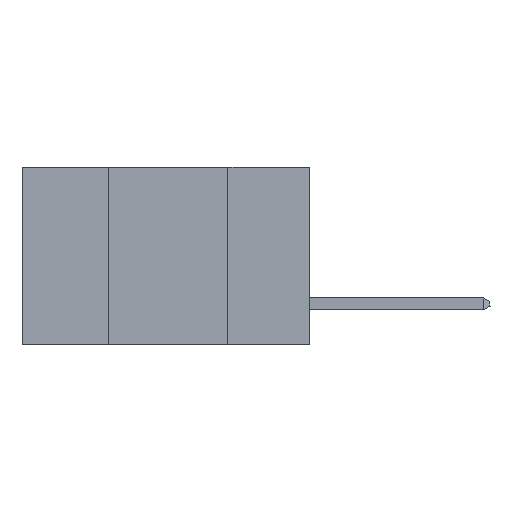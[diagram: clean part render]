
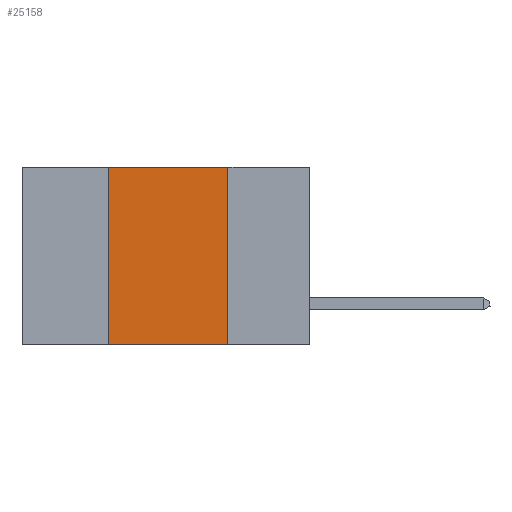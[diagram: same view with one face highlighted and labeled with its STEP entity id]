
A CAD part, left-side view. The second image highlights one B-rep face of the part: STEP entity #25158.
In plain terms, the highlighted planar face has unit normal (-1, 0, 0).
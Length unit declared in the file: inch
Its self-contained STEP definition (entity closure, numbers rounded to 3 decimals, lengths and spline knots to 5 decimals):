
#831 = DIRECTION ( 'NONE',  ( 0., 0., 1. ) ) ;
#963 = LINE ( 'NONE', #11146, #35582 ) ;
#2175 = ORIENTED_EDGE ( 'NONE', *, *, #39375, .F. ) ;
#4394 = EDGE_CURVE ( 'NONE', #23664, #35601, #20117, .T. ) ;
#5021 = ORIENTED_EDGE ( 'NONE', *, *, #14604, .F. ) ;
#5088 = PLANE ( 'NONE',  #15193 ) ;
#5428 = DIRECTION ( 'NONE',  ( 0., -1., 0. ) ) ;
#5784 = VECTOR ( 'NONE', #5428, 39.37008 ) ;
#6361 = EDGE_CURVE ( 'NONE', #16821, #35601, #38758, .T. ) ;
#9274 = DIRECTION ( 'NONE',  ( 0., -1., 0. ) ) ;
#10561 = FACE_OUTER_BOUND ( 'NONE', #16806, .T. ) ;
#11146 = CARTESIAN_POINT ( 'NONE',  ( 0., 0.42, 0. ) ) ;
#14604 = EDGE_CURVE ( 'NONE', #23664, #30111, #963, .T. ) ;
#15193 = AXIS2_PLACEMENT_3D ( 'NONE', #38428, #18243, #31505 ) ;
#16806 = EDGE_LOOP ( 'NONE', ( #23551, #2175, #5021, #19841 ) ) ;
#16821 = VERTEX_POINT ( 'NONE', #39368 ) ;
#16957 = VECTOR ( 'NONE', #9274, 39.37008 ) ;
#18243 = DIRECTION ( 'NONE',  ( 1., 0., 0. ) ) ;
#19841 = ORIENTED_EDGE ( 'NONE', *, *, #4394, .T. ) ;
#20117 = LINE ( 'NONE', #25928, #16957 ) ;
#23551 = ORIENTED_EDGE ( 'NONE', *, *, #6361, .F. ) ;
#23664 = VERTEX_POINT ( 'NONE', #42708 ) ;
#25158 = ADVANCED_FACE ( 'NONE', ( #10561 ), #5088, .F. ) ;
#25434 = CARTESIAN_POINT ( 'NONE',  ( 0., 0.6, 0. ) ) ;
#25928 = CARTESIAN_POINT ( 'NONE',  ( 0., 0.6, -0.37 ) ) ;
#30111 = VERTEX_POINT ( 'NONE', #32038 ) ;
#31505 = DIRECTION ( 'NONE',  ( 0., 0., -1. ) ) ;
#32038 = CARTESIAN_POINT ( 'NONE',  ( 0., 0.42, 0. ) ) ;
#35582 = VECTOR ( 'NONE', #831, 39.37008 ) ;
#35601 = VERTEX_POINT ( 'NONE', #38080 ) ;
#35967 = CARTESIAN_POINT ( 'NONE',  ( 0., 0.17, 0. ) ) ;
#38080 = CARTESIAN_POINT ( 'NONE',  ( 0., 0.17, -0.37 ) ) ;
#38428 = CARTESIAN_POINT ( 'NONE',  ( 0., 0.6, 0. ) ) ;
#38758 = LINE ( 'NONE', #35967, #40868 ) ;
#39304 = DIRECTION ( 'NONE',  ( 0., 0., -1. ) ) ;
#39368 = CARTESIAN_POINT ( 'NONE',  ( 0., 0.17, 0. ) ) ;
#39375 = EDGE_CURVE ( 'NONE', #30111, #16821, #41931, .T. ) ;
#40868 = VECTOR ( 'NONE', #39304, 39.37008 ) ;
#41931 = LINE ( 'NONE', #25434, #5784 ) ;
#42708 = CARTESIAN_POINT ( 'NONE',  ( 0., 0.42, -0.37 ) ) ;
